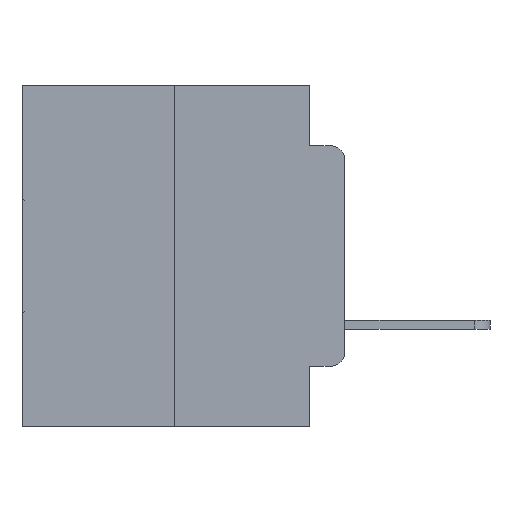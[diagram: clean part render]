
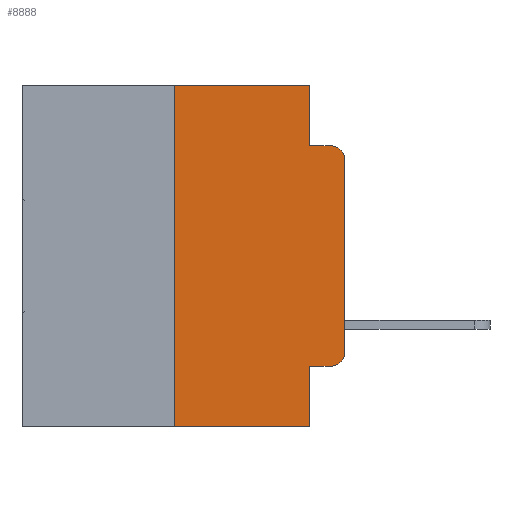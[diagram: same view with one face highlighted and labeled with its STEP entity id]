
A CAD part, left-side view. The second image highlights one B-rep face of the part: STEP entity #8888.
In plain terms, the highlighted planar face has unit normal (-1, 0, 0).
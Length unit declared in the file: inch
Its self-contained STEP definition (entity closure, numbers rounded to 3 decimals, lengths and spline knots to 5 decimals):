
#160 = DIRECTION ( 'NONE',  ( 0., 0., -1. ) ) ;
#546 = ORIENTED_EDGE ( 'NONE', *, *, #23519, .T. ) ;
#677 = CARTESIAN_POINT ( 'NONE',  ( 0., 0., -0.3915 ) ) ;
#1137 = DIRECTION ( 'NONE',  ( 0., -1., 0. ) ) ;
#1439 = CARTESIAN_POINT ( 'NONE',  ( 0., 0.25, -0.5 ) ) ;
#1571 = ORIENTED_EDGE ( 'NONE', *, *, #16982, .T. ) ;
#1757 = VERTEX_POINT ( 'NONE', #2997 ) ;
#2997 = CARTESIAN_POINT ( 'NONE',  ( 0., 0.25, 0. ) ) ;
#3044 = VERTEX_POINT ( 'NONE', #7618 ) ;
#3084 = ORIENTED_EDGE ( 'NONE', *, *, #6490, .T. ) ;
#3192 = DIRECTION ( 'NONE',  ( -1., 0., 0. ) ) ;
#3193 = VERTEX_POINT ( 'NONE', #677 ) ;
#3599 = CARTESIAN_POINT ( 'NONE',  ( 0., 0.051, -0.0885 ) ) ;
#4342 = VECTOR ( 'NONE', #25032, 39.37008 ) ;
#4748 = ORIENTED_EDGE ( 'NONE', *, *, #16082, .F. ) ;
#4776 = LINE ( 'NONE', #27501, #16607 ) ;
#4780 = PLANE ( 'NONE',  #24121 ) ;
#4879 = CARTESIAN_POINT ( 'NONE',  ( 0., 0.473, 0. ) ) ;
#6318 = EDGE_CURVE ( 'NONE', #9092, #9788, #25102, .T. ) ;
#6490 = EDGE_CURVE ( 'NONE', #3044, #17344, #14620, .T. ) ;
#6681 = DIRECTION ( 'NONE',  ( 0., 0., -1. ) ) ;
#6834 = ORIENTED_EDGE ( 'NONE', *, *, #18601, .T. ) ;
#6980 = VECTOR ( 'NONE', #21004, 39.37008 ) ;
#7618 = CARTESIAN_POINT ( 'NONE',  ( 0., 0., -0.1085 ) ) ;
#8537 = CARTESIAN_POINT ( 'NONE',  ( 0., 0.051, -0.4115 ) ) ;
#8812 = ORIENTED_EDGE ( 'NONE', *, *, #27937, .F. ) ;
#8860 = CIRCLE ( 'NONE', #18691, 0.02 ) ;
#8888 = ADVANCED_FACE ( 'NONE', ( #28167 ), #4780, .F. ) ;
#9092 = VERTEX_POINT ( 'NONE', #10148 ) ;
#9271 = VERTEX_POINT ( 'NONE', #17284 ) ;
#9788 = VERTEX_POINT ( 'NONE', #3599 ) ;
#9830 = CARTESIAN_POINT ( 'NONE',  ( 0., 0.473, -0.5 ) ) ;
#10148 = CARTESIAN_POINT ( 'NONE',  ( 0., 0.051, 0. ) ) ;
#10347 = VERTEX_POINT ( 'NONE', #1439 ) ;
#11058 = LINE ( 'NONE', #9830, #4342 ) ;
#11165 = DIRECTION ( 'NONE',  ( 0., 0., 1. ) ) ;
#11716 = EDGE_CURVE ( 'NONE', #9788, #17344, #13722, .T. ) ;
#12116 = CARTESIAN_POINT ( 'NONE',  ( 0., 0.02, -0.1085 ) ) ;
#12383 = VECTOR ( 'NONE', #13077, 39.37008 ) ;
#12736 = DIRECTION ( 'NONE',  ( 0., -1., 0. ) ) ;
#13047 = VECTOR ( 'NONE', #12736, 39.37008 ) ;
#13077 = DIRECTION ( 'NONE',  ( 0., 0., 1. ) ) ;
#13722 = LINE ( 'NONE', #14949, #13047 ) ;
#13813 = DIRECTION ( 'NONE',  ( 1., 0., 0. ) ) ;
#14341 = DIRECTION ( 'NONE',  ( 0., 0., -1. ) ) ;
#14620 = CIRCLE ( 'NONE', #23553, 0.02 ) ;
#14949 = CARTESIAN_POINT ( 'NONE',  ( 0., 0.051, -0.0885 ) ) ;
#15962 = VECTOR ( 'NONE', #11165, 39.37008 ) ;
#16082 = EDGE_CURVE ( 'NONE', #16594, #22306, #27478, .T. ) ;
#16127 = VECTOR ( 'NONE', #6681, 39.37008 ) ;
#16594 = VERTEX_POINT ( 'NONE', #8537 ) ;
#16606 = CARTESIAN_POINT ( 'NONE',  ( 0., 0.02, -0.3915 ) ) ;
#16607 = VECTOR ( 'NONE', #1137, 39.37008 ) ;
#16982 = EDGE_CURVE ( 'NONE', #9271, #3193, #8860, .T. ) ;
#17284 = CARTESIAN_POINT ( 'NONE',  ( 0., 0.02, -0.4115 ) ) ;
#17344 = VERTEX_POINT ( 'NONE', #19867 ) ;
#17432 = CARTESIAN_POINT ( 'NONE',  ( 0., 0.051, 0. ) ) ;
#17489 = LINE ( 'NONE', #23832, #12383 ) ;
#18486 = ORIENTED_EDGE ( 'NONE', *, *, #11716, .F. ) ;
#18601 = EDGE_CURVE ( 'NONE', #3193, #3044, #22345, .T. ) ;
#18691 = AXIS2_PLACEMENT_3D ( 'NONE', #16606, #3192, #18753 ) ;
#18753 = DIRECTION ( 'NONE',  ( 0., 0., -1. ) ) ;
#19867 = CARTESIAN_POINT ( 'NONE',  ( 0., 0.02, -0.0885 ) ) ;
#20158 = EDGE_CURVE ( 'NONE', #10347, #22306, #11058, .T. ) ;
#20301 = DIRECTION ( 'NONE',  ( 0., -1., 0. ) ) ;
#21004 = DIRECTION ( 'NONE',  ( 0., 0., -1. ) ) ;
#21024 = ORIENTED_EDGE ( 'NONE', *, *, #20158, .T. ) ;
#21507 = LINE ( 'NONE', #4879, #22863 ) ;
#22306 = VERTEX_POINT ( 'NONE', #24247 ) ;
#22345 = LINE ( 'NONE', #26313, #15962 ) ;
#22369 = CARTESIAN_POINT ( 'NONE',  ( 0., 0.473, 0. ) ) ;
#22756 = ORIENTED_EDGE ( 'NONE', *, *, #27711, .F. ) ;
#22863 = VECTOR ( 'NONE', #20301, 39.37008 ) ;
#23519 = EDGE_CURVE ( 'NONE', #16594, #9271, #4776, .T. ) ;
#23553 = AXIS2_PLACEMENT_3D ( 'NONE', #12116, #27158, #14341 ) ;
#23832 = CARTESIAN_POINT ( 'NONE',  ( 0., 0.25, 0. ) ) ;
#23913 = ORIENTED_EDGE ( 'NONE', *, *, #6318, .F. ) ;
#24121 = AXIS2_PLACEMENT_3D ( 'NONE', #22369, #13813, #160 ) ;
#24149 = CARTESIAN_POINT ( 'NONE',  ( 0., 0.051, 0. ) ) ;
#24247 = CARTESIAN_POINT ( 'NONE',  ( 0., 0.051, -0.5 ) ) ;
#25032 = DIRECTION ( 'NONE',  ( 0., -1., 0. ) ) ;
#25102 = LINE ( 'NONE', #17432, #6980 ) ;
#26313 = CARTESIAN_POINT ( 'NONE',  ( 0., 0., 0. ) ) ;
#27158 = DIRECTION ( 'NONE',  ( -1., 0., 0. ) ) ;
#27478 = LINE ( 'NONE', #24149, #16127 ) ;
#27501 = CARTESIAN_POINT ( 'NONE',  ( 0., 0.051, -0.4115 ) ) ;
#27711 = EDGE_CURVE ( 'NONE', #10347, #1757, #17489, .T. ) ;
#27937 = EDGE_CURVE ( 'NONE', #1757, #9092, #21507, .T. ) ;
#28167 = FACE_OUTER_BOUND ( 'NONE', #28244, .T. ) ;
#28244 = EDGE_LOOP ( 'NONE', ( #6834, #3084, #18486, #23913, #8812, #22756, #21024, #4748, #546, #1571 ) ) ;
